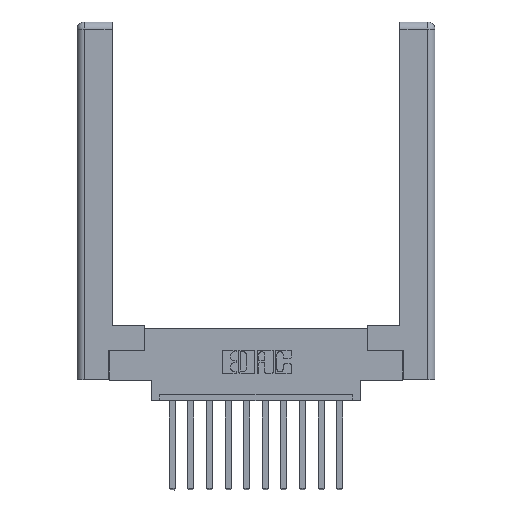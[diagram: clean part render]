
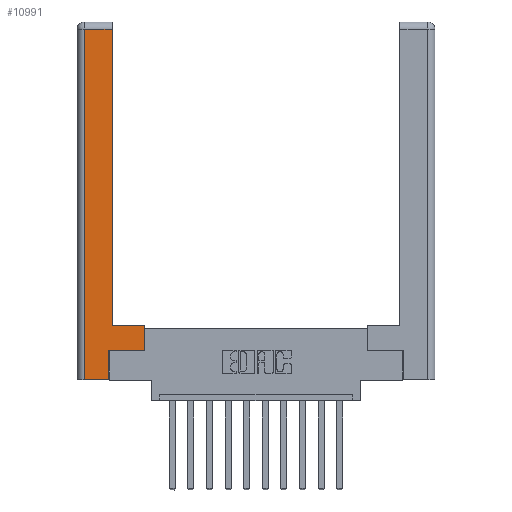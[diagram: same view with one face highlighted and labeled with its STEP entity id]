
A CAD part, top view. The second image highlights one B-rep face of the part: STEP entity #10991.
In plain terms, the highlighted planar face has unit normal (0, 0, 1).
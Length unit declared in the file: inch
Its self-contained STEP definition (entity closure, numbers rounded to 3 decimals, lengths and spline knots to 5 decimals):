
#791 = CARTESIAN_POINT ( 'NONE',  ( 0.0615, 0., 0. ) ) ;
#904 = EDGE_CURVE ( 'NONE', #2498, #10588, #6487, .T. ) ;
#1138 = CARTESIAN_POINT ( 'NONE',  ( 0.295, 0.45, 0. ) ) ;
#1288 = ORIENTED_EDGE ( 'NONE', *, *, #6282, .T. ) ;
#1420 = EDGE_CURVE ( 'NONE', #5012, #1426, #12235, .T. ) ;
#1426 = VERTEX_POINT ( 'NONE', #5614 ) ;
#1479 = DIRECTION ( 'NONE',  ( -1., 0., 0. ) ) ;
#2041 = ORIENTED_EDGE ( 'NONE', *, *, #1420, .T. ) ;
#2358 = CARTESIAN_POINT ( 'NONE',  ( 0.0615, 2.94, 0. ) ) ;
#2498 = VERTEX_POINT ( 'NONE', #4963 ) ;
#3059 = CARTESIAN_POINT ( 'NONE',  ( 0.0615, 0., 0. ) ) ;
#3145 = EDGE_CURVE ( 'NONE', #11846, #3221, #3437, .T. ) ;
#3146 = LINE ( 'NONE', #14076, #9509 ) ;
#3166 = LINE ( 'NONE', #6920, #11561 ) ;
#3221 = VERTEX_POINT ( 'NONE', #3059 ) ;
#3314 = DIRECTION ( 'NONE',  ( -1., 0., 0. ) ) ;
#3437 = LINE ( 'NONE', #791, #4314 ) ;
#3519 = LINE ( 'NONE', #6121, #6127 ) ;
#3700 = DIRECTION ( 'NONE',  ( 0., 1., 0. ) ) ;
#3711 = PLANE ( 'NONE',  #11853 ) ;
#3974 = CARTESIAN_POINT ( 'NONE',  ( 0.295, 2.94, 0. ) ) ;
#4040 = ORIENTED_EDGE ( 'NONE', *, *, #3145, .T. ) ;
#4314 = VECTOR ( 'NONE', #12838, 39.37008 ) ;
#4422 = ORIENTED_EDGE ( 'NONE', *, *, #6987, .T. ) ;
#4963 = CARTESIAN_POINT ( 'NONE',  ( 0.265, 0.245, 0. ) ) ;
#5012 = VERTEX_POINT ( 'NONE', #6982 ) ;
#5457 = EDGE_LOOP ( 'NONE', ( #6219, #4422, #4040, #11394, #11620, #12896, #1288, #2041 ) ) ;
#5614 = CARTESIAN_POINT ( 'NONE',  ( 0.295, 0.45, 0. ) ) ;
#5824 = CARTESIAN_POINT ( 'NONE',  ( 0.265, 0., 0. ) ) ;
#6121 = CARTESIAN_POINT ( 'NONE',  ( 0.565, 0.45, 0. ) ) ;
#6127 = VECTOR ( 'NONE', #3700, 39.37008 ) ;
#6219 = ORIENTED_EDGE ( 'NONE', *, *, #9137, .T. ) ;
#6282 = EDGE_CURVE ( 'NONE', #10588, #5012, #3519, .T. ) ;
#6289 = CARTESIAN_POINT ( 'NONE',  ( 0.565, 0.245, 0. ) ) ;
#6487 = LINE ( 'NONE', #6289, #6663 ) ;
#6520 = VERTEX_POINT ( 'NONE', #5824 ) ;
#6663 = VECTOR ( 'NONE', #8035, 39.37008 ) ;
#6748 = CARTESIAN_POINT ( 'NONE',  ( 0.295, 3., 0. ) ) ;
#6799 = VERTEX_POINT ( 'NONE', #3974 ) ;
#6885 = DIRECTION ( 'NONE',  ( 0., 1., 0. ) ) ;
#6904 = EDGE_CURVE ( 'NONE', #3221, #6520, #7802, .T. ) ;
#6920 = CARTESIAN_POINT ( 'NONE',  ( 0.0615, 2.94, 0. ) ) ;
#6982 = CARTESIAN_POINT ( 'NONE',  ( 0.565, 0.45, 0. ) ) ;
#6987 = EDGE_CURVE ( 'NONE', #6799, #11846, #3166, .T. ) ;
#7648 = DIRECTION ( 'NONE',  ( 1., 0., 0. ) ) ;
#7802 = LINE ( 'NONE', #13109, #13792 ) ;
#7967 = DIRECTION ( 'NONE',  ( -1., 0., 0. ) ) ;
#8035 = DIRECTION ( 'NONE',  ( 1., 0., 0. ) ) ;
#9137 = EDGE_CURVE ( 'NONE', #1426, #6799, #11546, .T. ) ;
#9509 = VECTOR ( 'NONE', #9777, 39.37008 ) ;
#9777 = DIRECTION ( 'NONE',  ( 0., 1., 0. ) ) ;
#9879 = VECTOR ( 'NONE', #3314, 39.37008 ) ;
#9882 = EDGE_CURVE ( 'NONE', #6520, #2498, #3146, .T. ) ;
#10127 = DIRECTION ( 'NONE',  ( 0., 0., -1. ) ) ;
#10375 = VECTOR ( 'NONE', #6885, 39.37008 ) ;
#10588 = VERTEX_POINT ( 'NONE', #13021 ) ;
#10991 = ADVANCED_FACE ( 'NONE', ( #13592 ), #3711, .F. ) ;
#11175 = CARTESIAN_POINT ( 'NONE',  ( 0., 0., 0. ) ) ;
#11394 = ORIENTED_EDGE ( 'NONE', *, *, #6904, .T. ) ;
#11546 = LINE ( 'NONE', #6748, #10375 ) ;
#11561 = VECTOR ( 'NONE', #7967, 39.37008 ) ;
#11620 = ORIENTED_EDGE ( 'NONE', *, *, #9882, .T. ) ;
#11846 = VERTEX_POINT ( 'NONE', #2358 ) ;
#11853 = AXIS2_PLACEMENT_3D ( 'NONE', #11175, #10127, #1479 ) ;
#12235 = LINE ( 'NONE', #1138, #9879 ) ;
#12838 = DIRECTION ( 'NONE',  ( 0., -1., 0. ) ) ;
#12896 = ORIENTED_EDGE ( 'NONE', *, *, #904, .T. ) ;
#13021 = CARTESIAN_POINT ( 'NONE',  ( 0.565, 0.245, 0. ) ) ;
#13109 = CARTESIAN_POINT ( 'NONE',  ( 0.265, 0., 0. ) ) ;
#13592 = FACE_OUTER_BOUND ( 'NONE', #5457, .T. ) ;
#13792 = VECTOR ( 'NONE', #7648, 39.37008 ) ;
#14076 = CARTESIAN_POINT ( 'NONE',  ( 0.265, 0.245, 0. ) ) ;
